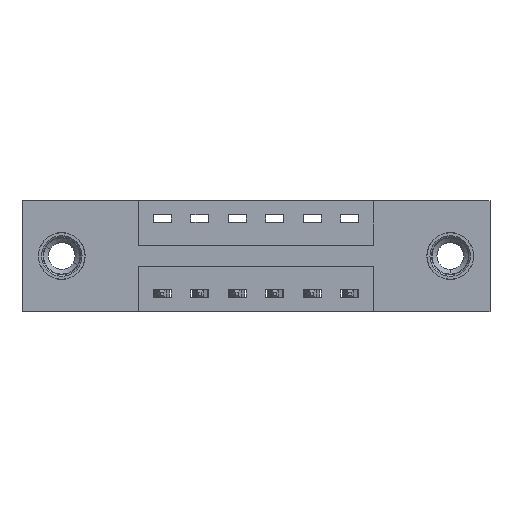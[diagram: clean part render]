
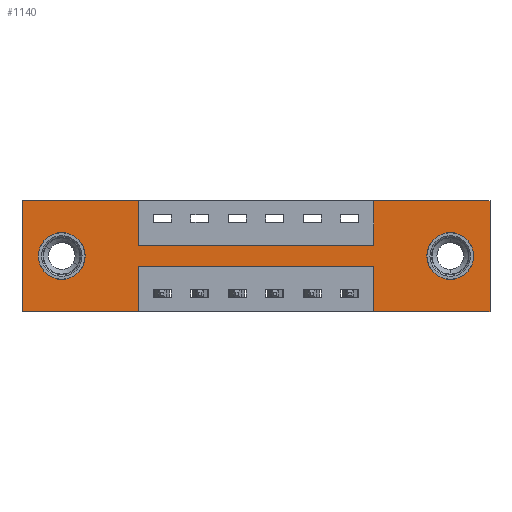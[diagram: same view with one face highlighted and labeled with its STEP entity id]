
A CAD part, front view. The second image highlights one B-rep face of the part: STEP entity #1140.
In plain terms, the highlighted planar face has unit normal (0, -1, 0).
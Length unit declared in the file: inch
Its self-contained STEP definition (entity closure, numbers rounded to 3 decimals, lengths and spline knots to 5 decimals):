
#3 = CARTESIAN_POINT ( 'NONE',  ( 1.4275, 0., -0.107 ) ) ;
#17 = CARTESIAN_POINT ( 'NONE',  ( 1.1725, 0., 0. ) ) ;
#182 = EDGE_CURVE ( 'NONE', #3551, #1499, #321, .T. ) ;
#205 = EDGE_CURVE ( 'NONE', #1583, #8474, #4071, .T. ) ;
#217 = CARTESIAN_POINT ( 'NONE',  ( 0.1325, 0., -0.107 ) ) ;
#321 = CIRCLE ( 'NONE', #5085, 0.078 ) ;
#340 = VERTEX_POINT ( 'NONE', #873 ) ;
#380 = DIRECTION ( 'NONE',  ( 0., 0., 1. ) ) ;
#386 = DIRECTION ( 'NONE',  ( 0., 0., -1. ) ) ;
#412 = DIRECTION ( 'NONE',  ( -1., 0., 0. ) ) ;
#442 = EDGE_CURVE ( 'NONE', #1499, #3551, #7995, .T. ) ;
#520 = ORIENTED_EDGE ( 'NONE', *, *, #7503, .F. ) ;
#586 = LINE ( 'NONE', #1861, #8372 ) ;
#610 = ORIENTED_EDGE ( 'NONE', *, *, #2204, .F. ) ;
#625 = CARTESIAN_POINT ( 'NONE',  ( 1.4275, 0., -0.263 ) ) ;
#873 = CARTESIAN_POINT ( 'NONE',  ( 0., 0., -0.37 ) ) ;
#948 = VERTEX_POINT ( 'NONE', #4207 ) ;
#968 = CIRCLE ( 'NONE', #6236, 0.078 ) ;
#1067 = VECTOR ( 'NONE', #5160, 39.37008 ) ;
#1133 = CARTESIAN_POINT ( 'NONE',  ( 0., 0., 0. ) ) ;
#1140 = ADVANCED_FACE ( 'NONE', ( #9637, #7366, #3596 ), #6788, .T. ) ;
#1218 = CARTESIAN_POINT ( 'NONE',  ( 1.1725, 0., -0.37 ) ) ;
#1262 = CARTESIAN_POINT ( 'NONE',  ( 0.1325, 0., -0.185 ) ) ;
#1400 = AXIS2_PLACEMENT_3D ( 'NONE', #1262, #1490, #6107 ) ;
#1490 = DIRECTION ( 'NONE',  ( 0., 1., 0. ) ) ;
#1499 = VERTEX_POINT ( 'NONE', #217 ) ;
#1525 = CARTESIAN_POINT ( 'NONE',  ( 0.3875, 0., -0.15 ) ) ;
#1558 = DIRECTION ( 'NONE',  ( 0., 0., -1. ) ) ;
#1578 = CARTESIAN_POINT ( 'NONE',  ( 1.4275, 0., -0.185 ) ) ;
#1583 = VERTEX_POINT ( 'NONE', #6359 ) ;
#1651 = CARTESIAN_POINT ( 'NONE',  ( 0.3875, 0., -0.22 ) ) ;
#1663 = VERTEX_POINT ( 'NONE', #1133 ) ;
#1749 = CARTESIAN_POINT ( 'NONE',  ( 1.56, 0., 0. ) ) ;
#1817 = VECTOR ( 'NONE', #380, 39.37008 ) ;
#1861 = CARTESIAN_POINT ( 'NONE',  ( 0., 0., -0.37 ) ) ;
#1867 = VECTOR ( 'NONE', #3283, 39.37008 ) ;
#1873 = EDGE_CURVE ( 'NONE', #3295, #6513, #2507, .T. ) ;
#2158 = CARTESIAN_POINT ( 'NONE',  ( 0.3875, 0., -0.37 ) ) ;
#2204 = EDGE_CURVE ( 'NONE', #4212, #948, #6090, .T. ) ;
#2244 = ORIENTED_EDGE ( 'NONE', *, *, #442, .T. ) ;
#2254 = ORIENTED_EDGE ( 'NONE', *, *, #6006, .F. ) ;
#2331 = DIRECTION ( 'NONE',  ( 0., 0., -1. ) ) ;
#2476 = VERTEX_POINT ( 'NONE', #3 ) ;
#2507 = LINE ( 'NONE', #2158, #2741 ) ;
#2539 = VERTEX_POINT ( 'NONE', #9123 ) ;
#2597 = ORIENTED_EDGE ( 'NONE', *, *, #7379, .F. ) ;
#2709 = VERTEX_POINT ( 'NONE', #1749 ) ;
#2733 = CARTESIAN_POINT ( 'NONE',  ( 1.4275, 0., -0.185 ) ) ;
#2737 = CARTESIAN_POINT ( 'NONE',  ( 0.1325, 0., -0.263 ) ) ;
#2741 = VECTOR ( 'NONE', #7459, 39.37008 ) ;
#2759 = DIRECTION ( 'NONE',  ( 1., 0., 0. ) ) ;
#2856 = ORIENTED_EDGE ( 'NONE', *, *, #205, .F. ) ;
#3065 = VECTOR ( 'NONE', #6647, 39.37008 ) ;
#3095 = EDGE_LOOP ( 'NONE', ( #9001, #2597, #610, #4138, #2254, #6625, #2856, #9448, #6281, #4961, #520, #8980 ) ) ;
#3283 = DIRECTION ( 'NONE',  ( 0., 0., -1. ) ) ;
#3295 = VERTEX_POINT ( 'NONE', #1651 ) ;
#3495 = VECTOR ( 'NONE', #1558, 39.37008 ) ;
#3496 = DIRECTION ( 'NONE',  ( 0., 0., 1. ) ) ;
#3499 = DIRECTION ( 'NONE',  ( 0., 0., -1. ) ) ;
#3551 = VERTEX_POINT ( 'NONE', #2737 ) ;
#3596 = FACE_OUTER_BOUND ( 'NONE', #3095, .T. ) ;
#3663 = LINE ( 'NONE', #7804, #1867 ) ;
#4039 = DIRECTION ( 'NONE',  ( 0., 0., 1. ) ) ;
#4063 = VECTOR ( 'NONE', #3496, 39.37008 ) ;
#4071 = LINE ( 'NONE', #17, #1817 ) ;
#4138 = ORIENTED_EDGE ( 'NONE', *, *, #5134, .F. ) ;
#4207 = CARTESIAN_POINT ( 'NONE',  ( 1.1725, 0., -0.22 ) ) ;
#4212 = VERTEX_POINT ( 'NONE', #9579 ) ;
#4671 = CARTESIAN_POINT ( 'NONE',  ( 0., 0., -0.37 ) ) ;
#4718 = DIRECTION ( 'NONE',  ( 0., -1., 0. ) ) ;
#4762 = ORIENTED_EDGE ( 'NONE', *, *, #182, .T. ) ;
#4873 = CARTESIAN_POINT ( 'NONE',  ( 0.3875, 0., -0.15 ) ) ;
#4961 = ORIENTED_EDGE ( 'NONE', *, *, #5117, .F. ) ;
#5085 = AXIS2_PLACEMENT_3D ( 'NONE', #6242, #9740, #8222 ) ;
#5117 = EDGE_CURVE ( 'NONE', #1663, #6727, #7089, .T. ) ;
#5134 = EDGE_CURVE ( 'NONE', #2539, #4212, #8865, .T. ) ;
#5160 = DIRECTION ( 'NONE',  ( -1., 0., 0. ) ) ;
#5617 = CARTESIAN_POINT ( 'NONE',  ( 0.3875, 0., 0. ) ) ;
#5759 = LINE ( 'NONE', #7053, #7512 ) ;
#5829 = EDGE_LOOP ( 'NONE', ( #9612, #6866 ) ) ;
#5869 = CARTESIAN_POINT ( 'NONE',  ( 0., 0., 0. ) ) ;
#6006 = EDGE_CURVE ( 'NONE', #2709, #2539, #3663, .T. ) ;
#6090 = LINE ( 'NONE', #1218, #4063 ) ;
#6093 = CARTESIAN_POINT ( 'NONE',  ( 0.3875, 0., 0. ) ) ;
#6107 = DIRECTION ( 'NONE',  ( 0., 0., 1. ) ) ;
#6236 = AXIS2_PLACEMENT_3D ( 'NONE', #1578, #6873, #2331 ) ;
#6242 = CARTESIAN_POINT ( 'NONE',  ( 0.1325, 0., -0.185 ) ) ;
#6281 = ORIENTED_EDGE ( 'NONE', *, *, #7990, .F. ) ;
#6359 = CARTESIAN_POINT ( 'NONE',  ( 1.1725, 0., -0.15 ) ) ;
#6424 = AXIS2_PLACEMENT_3D ( 'NONE', #2733, #8041, #3499 ) ;
#6458 = VERTEX_POINT ( 'NONE', #1525 ) ;
#6513 = VERTEX_POINT ( 'NONE', #7624 ) ;
#6606 = AXIS2_PLACEMENT_3D ( 'NONE', #4671, #4718, #386 ) ;
#6625 = ORIENTED_EDGE ( 'NONE', *, *, #6893, .F. ) ;
#6647 = DIRECTION ( 'NONE',  ( 1., 0., 0. ) ) ;
#6653 = CARTESIAN_POINT ( 'NONE',  ( 1.1725, 0., 0. ) ) ;
#6727 = VERTEX_POINT ( 'NONE', #5617 ) ;
#6737 = VECTOR ( 'NONE', #7144, 39.37008 ) ;
#6785 = EDGE_CURVE ( 'NONE', #6513, #340, #586, .T. ) ;
#6788 = PLANE ( 'NONE',  #6606 ) ;
#6866 = ORIENTED_EDGE ( 'NONE', *, *, #8346, .T. ) ;
#6873 = DIRECTION ( 'NONE',  ( 0., 1., 0. ) ) ;
#6893 = EDGE_CURVE ( 'NONE', #8474, #2709, #9680, .T. ) ;
#6947 = LINE ( 'NONE', #8380, #8710 ) ;
#6973 = LINE ( 'NONE', #4873, #6737 ) ;
#7053 = CARTESIAN_POINT ( 'NONE',  ( 0., 0., 0. ) ) ;
#7089 = LINE ( 'NONE', #5869, #3065 ) ;
#7144 = DIRECTION ( 'NONE',  ( 1., 0., 0. ) ) ;
#7250 = CARTESIAN_POINT ( 'NONE',  ( 0., 0., 0. ) ) ;
#7366 = FACE_BOUND ( 'NONE', #9255, .T. ) ;
#7379 = EDGE_CURVE ( 'NONE', #948, #3295, #6947, .T. ) ;
#7459 = DIRECTION ( 'NONE',  ( 0., 0., -1. ) ) ;
#7503 = EDGE_CURVE ( 'NONE', #340, #1663, #5759, .T. ) ;
#7512 = VECTOR ( 'NONE', #4039, 39.37008 ) ;
#7624 = CARTESIAN_POINT ( 'NONE',  ( 0.3875, 0., -0.37 ) ) ;
#7649 = VECTOR ( 'NONE', #2759, 39.37008 ) ;
#7804 = CARTESIAN_POINT ( 'NONE',  ( 1.56, 0., 0. ) ) ;
#7990 = EDGE_CURVE ( 'NONE', #6727, #6458, #9296, .T. ) ;
#7995 = CIRCLE ( 'NONE', #1400, 0.078 ) ;
#8041 = DIRECTION ( 'NONE',  ( 0., 1., 0. ) ) ;
#8222 = DIRECTION ( 'NONE',  ( 0., 0., 1. ) ) ;
#8346 = EDGE_CURVE ( 'NONE', #9614, #2476, #9352, .T. ) ;
#8372 = VECTOR ( 'NONE', #412, 39.37008 ) ;
#8380 = CARTESIAN_POINT ( 'NONE',  ( 0.3875, 0., -0.22 ) ) ;
#8448 = DIRECTION ( 'NONE',  ( -1., 0., 0. ) ) ;
#8474 = VERTEX_POINT ( 'NONE', #6653 ) ;
#8667 = EDGE_CURVE ( 'NONE', #2476, #9614, #968, .T. ) ;
#8710 = VECTOR ( 'NONE', #8448, 39.37008 ) ;
#8865 = LINE ( 'NONE', #9683, #1067 ) ;
#8980 = ORIENTED_EDGE ( 'NONE', *, *, #6785, .F. ) ;
#9001 = ORIENTED_EDGE ( 'NONE', *, *, #1873, .F. ) ;
#9123 = CARTESIAN_POINT ( 'NONE',  ( 1.56, 0., -0.37 ) ) ;
#9255 = EDGE_LOOP ( 'NONE', ( #2244, #4762 ) ) ;
#9296 = LINE ( 'NONE', #6093, #3495 ) ;
#9352 = CIRCLE ( 'NONE', #6424, 0.078 ) ;
#9448 = ORIENTED_EDGE ( 'NONE', *, *, #9506, .F. ) ;
#9506 = EDGE_CURVE ( 'NONE', #6458, #1583, #6973, .T. ) ;
#9579 = CARTESIAN_POINT ( 'NONE',  ( 1.1725, 0., -0.37 ) ) ;
#9612 = ORIENTED_EDGE ( 'NONE', *, *, #8667, .T. ) ;
#9614 = VERTEX_POINT ( 'NONE', #625 ) ;
#9637 = FACE_BOUND ( 'NONE', #5829, .T. ) ;
#9680 = LINE ( 'NONE', #7250, #7649 ) ;
#9683 = CARTESIAN_POINT ( 'NONE',  ( 0., 0., -0.37 ) ) ;
#9740 = DIRECTION ( 'NONE',  ( 0., 1., 0. ) ) ;
